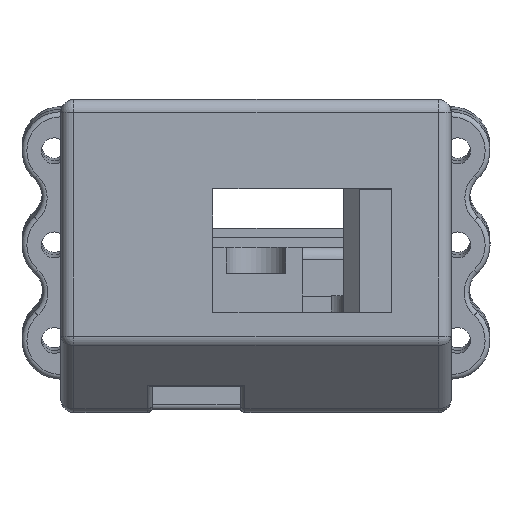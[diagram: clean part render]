
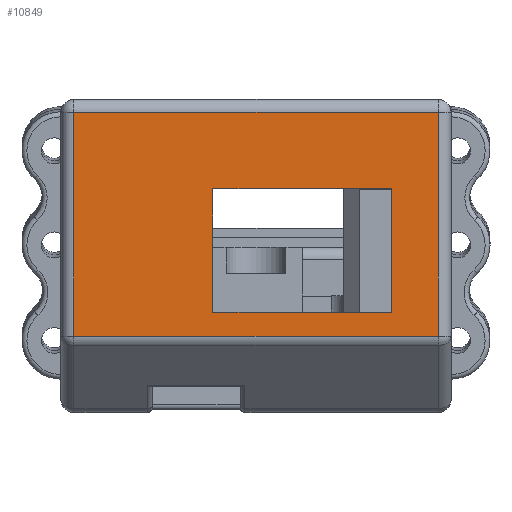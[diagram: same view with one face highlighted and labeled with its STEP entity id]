
A CAD part, top view. The second image highlights one B-rep face of the part: STEP entity #10849.
In plain terms, the highlighted planar face has unit normal (0, 0, 1).
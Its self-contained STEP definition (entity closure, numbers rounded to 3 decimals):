
#441=FACE_BOUND('',#1866,.T.);
#703=PLANE('',#11892);
#1156=FACE_OUTER_BOUND('',#1865,.T.);
#1865=EDGE_LOOP('',(#9151,#9152,#9153,#9154));
#1866=EDGE_LOOP('',(#9155,#9156,#9157,#9158));
#2787=LINE('',#19249,#3640);
#2819=LINE('',#19319,#3672);
#2821=LINE('',#19324,#3674);
#2822=LINE('',#19326,#3675);
#2823=LINE('',#19328,#3676);
#2824=LINE('',#19329,#3677);
#2825=LINE('',#19330,#3678);
#2826=LINE('',#19331,#3679);
#3640=VECTOR('',#14430,10.);
#3672=VECTOR('',#14486,10.);
#3674=VECTOR('',#14490,10.);
#3675=VECTOR('',#14491,10.);
#3676=VECTOR('',#14492,10.);
#3677=VECTOR('',#14493,10.);
#3678=VECTOR('',#14494,10.);
#3679=VECTOR('',#14495,10.);
#5131=VERTEX_POINT('',#19246);
#5132=VERTEX_POINT('',#19248);
#5157=VERTEX_POINT('',#19316);
#5158=VERTEX_POINT('',#19318);
#5159=VERTEX_POINT('',#19322);
#5160=VERTEX_POINT('',#19323);
#5161=VERTEX_POINT('',#19325);
#5162=VERTEX_POINT('',#19327);
#6513=EDGE_CURVE('',#5132,#5131,#2787,.T.);
#6549=EDGE_CURVE('',#5158,#5157,#2819,.T.);
#6551=EDGE_CURVE('',#5159,#5160,#2821,.T.);
#6552=EDGE_CURVE('',#5161,#5159,#2822,.T.);
#6553=EDGE_CURVE('',#5162,#5161,#2823,.T.);
#6554=EDGE_CURVE('',#5160,#5162,#2824,.T.);
#6555=EDGE_CURVE('',#5131,#5158,#2825,.T.);
#6556=EDGE_CURVE('',#5157,#5132,#2826,.T.);
#9151=ORIENTED_EDGE('',*,*,#6551,.F.);
#9152=ORIENTED_EDGE('',*,*,#6552,.F.);
#9153=ORIENTED_EDGE('',*,*,#6553,.F.);
#9154=ORIENTED_EDGE('',*,*,#6554,.F.);
#9155=ORIENTED_EDGE('',*,*,#6555,.T.);
#9156=ORIENTED_EDGE('',*,*,#6549,.T.);
#9157=ORIENTED_EDGE('',*,*,#6556,.T.);
#9158=ORIENTED_EDGE('',*,*,#6513,.T.);
#10849=ADVANCED_FACE('',(#1156,#441),#703,.T.);
#11892=AXIS2_PLACEMENT_3D('',#19321,#14488,#14489);
#14430=DIRECTION('',(1.,0.,0.));
#14486=DIRECTION('',(-1.,0.,0.));
#14488=DIRECTION('center_axis',(0.,0.,1.));
#14489=DIRECTION('ref_axis',(1.,0.,0.));
#14490=DIRECTION('',(-1.,0.,0.));
#14491=DIRECTION('',(0.,-1.,0.));
#14492=DIRECTION('',(1.,0.,0.));
#14493=DIRECTION('',(0.,1.,0.));
#14494=DIRECTION('',(0.,-1.,0.));
#14495=DIRECTION('',(0.,1.,0.));
#19246=CARTESIAN_POINT('',(20.956,-13.887,267.));
#19248=CARTESIAN_POINT('',(-6.656,-13.887,267.));
#19249=CARTESIAN_POINT('',(-6.656,-13.887,267.));
#19316=CARTESIAN_POINT('',(-6.656,-32.934,267.));
#19318=CARTESIAN_POINT('',(20.956,-32.934,267.));
#19319=CARTESIAN_POINT('',(10.478,-32.934,267.));
#19321=CARTESIAN_POINT('Origin',(0.,-24.313,267.));
#19322=CARTESIAN_POINT('',(28.1,-36.614,267.));
#19323=CARTESIAN_POINT('',(-28.1,-36.614,267.));
#19324=CARTESIAN_POINT('',(5.8,-36.614,267.));
#19325=CARTESIAN_POINT('',(28.1,-2.086,267.));
#19326=CARTESIAN_POINT('',(28.1,-24.313,267.));
#19327=CARTESIAN_POINT('',(-28.1,-2.086,267.));
#19328=CARTESIAN_POINT('',(8.05,-2.086,267.));
#19329=CARTESIAN_POINT('',(-28.1,-24.313,267.));
#19330=CARTESIAN_POINT('',(20.956,-0.086,267.));
#19331=CARTESIAN_POINT('',(-6.656,-32.055,267.));
